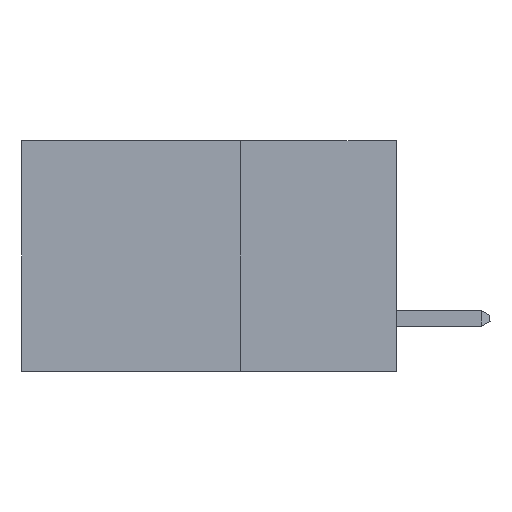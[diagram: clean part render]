
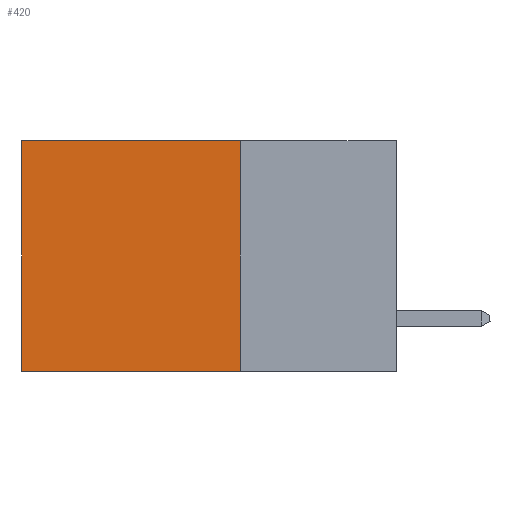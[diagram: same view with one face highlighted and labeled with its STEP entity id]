
A CAD part, left-side view. The second image highlights one B-rep face of the part: STEP entity #420.
In plain terms, the highlighted planar face has unit normal (-1, 0, 0).
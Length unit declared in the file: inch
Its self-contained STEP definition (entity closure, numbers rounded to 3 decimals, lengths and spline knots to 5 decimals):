
#420 = ADVANCED_FACE ( 'NONE', ( #15650 ), #915, .F. ) ;
#608 = LINE ( 'NONE', #12261, #10587 ) ;
#683 = DIRECTION ( 'NONE',  ( 0., 1., 0. ) ) ;
#915 = PLANE ( 'NONE',  #14580 ) ;
#1215 = CARTESIAN_POINT ( 'NONE',  ( 0.298, 0.25, 0. ) ) ;
#1427 = DIRECTION ( 'NONE',  ( 0., 0., -1. ) ) ;
#1616 = VERTEX_POINT ( 'NONE', #16031 ) ;
#1979 = CARTESIAN_POINT ( 'NONE',  ( 0.298, 0.6, -0.37 ) ) ;
#2356 = ORIENTED_EDGE ( 'NONE', *, *, #2918, .T. ) ;
#2416 = DIRECTION ( 'NONE',  ( 1., 0., 0. ) ) ;
#2918 = EDGE_CURVE ( 'NONE', #11187, #1616, #6203, .T. ) ;
#3162 = DIRECTION ( 'NONE',  ( 0., 0., -1. ) ) ;
#3256 = CARTESIAN_POINT ( 'NONE',  ( 0.298, 0.25, -0.37 ) ) ;
#3265 = ORIENTED_EDGE ( 'NONE', *, *, #6479, .F. ) ;
#3503 = LINE ( 'NONE', #13517, #13037 ) ;
#4555 = DIRECTION ( 'NONE',  ( 0., 0., -1. ) ) ;
#6203 = LINE ( 'NONE', #13023, #9655 ) ;
#6479 = EDGE_CURVE ( 'NONE', #13443, #14091, #7485, .T. ) ;
#7485 = LINE ( 'NONE', #3256, #10508 ) ;
#8140 = CARTESIAN_POINT ( 'NONE',  ( 0.298, 0.25, 0. ) ) ;
#9655 = VECTOR ( 'NONE', #14873, 39.37008 ) ;
#10508 = VECTOR ( 'NONE', #683, 39.37008 ) ;
#10587 = VECTOR ( 'NONE', #4555, 39.37008 ) ;
#10665 = EDGE_LOOP ( 'NONE', ( #13805, #3265, #12538, #2356 ) ) ;
#11187 = VERTEX_POINT ( 'NONE', #1215 ) ;
#11368 = EDGE_CURVE ( 'NONE', #11187, #13443, #3503, .T. ) ;
#12261 = CARTESIAN_POINT ( 'NONE',  ( 0.298, 0.6, 0. ) ) ;
#12538 = ORIENTED_EDGE ( 'NONE', *, *, #11368, .F. ) ;
#13023 = CARTESIAN_POINT ( 'NONE',  ( 0.298, 0.25, 0. ) ) ;
#13037 = VECTOR ( 'NONE', #3162, 39.37008 ) ;
#13406 = EDGE_CURVE ( 'NONE', #1616, #14091, #608, .T. ) ;
#13443 = VERTEX_POINT ( 'NONE', #14773 ) ;
#13517 = CARTESIAN_POINT ( 'NONE',  ( 0.298, 0.25, 0. ) ) ;
#13805 = ORIENTED_EDGE ( 'NONE', *, *, #13406, .T. ) ;
#14091 = VERTEX_POINT ( 'NONE', #1979 ) ;
#14580 = AXIS2_PLACEMENT_3D ( 'NONE', #8140, #2416, #1427 ) ;
#14773 = CARTESIAN_POINT ( 'NONE',  ( 0.298, 0.25, -0.37 ) ) ;
#14873 = DIRECTION ( 'NONE',  ( 0., 1., 0. ) ) ;
#15650 = FACE_OUTER_BOUND ( 'NONE', #10665, .T. ) ;
#16031 = CARTESIAN_POINT ( 'NONE',  ( 0.298, 0.6, 0. ) ) ;
